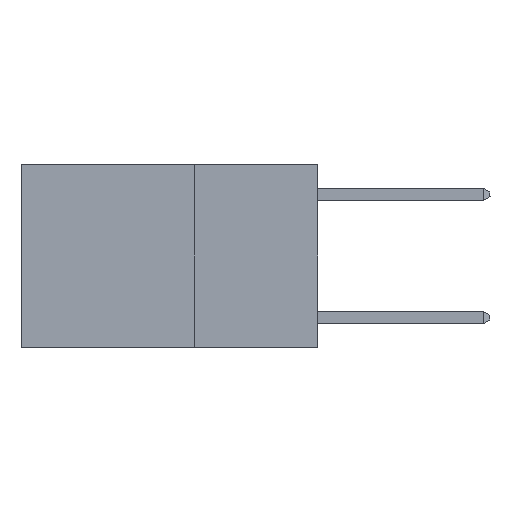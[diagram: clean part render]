
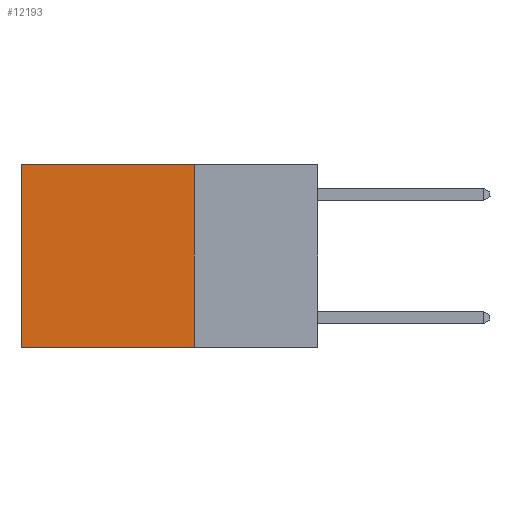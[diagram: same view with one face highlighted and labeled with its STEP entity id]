
A CAD part, left-side view. The second image highlights one B-rep face of the part: STEP entity #12193.
In plain terms, the highlighted planar face has unit normal (-1, 0, 0).
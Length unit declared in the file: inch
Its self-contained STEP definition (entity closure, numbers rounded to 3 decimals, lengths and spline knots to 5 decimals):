
#111 = LINE ( 'NONE', #9162, #2902 ) ;
#251 = VERTEX_POINT ( 'NONE', #11108 ) ;
#793 = CARTESIAN_POINT ( 'NONE',  ( 0.2625, 0.6, -0.37 ) ) ;
#811 = EDGE_CURVE ( 'NONE', #4362, #7198, #11759, .T. ) ;
#1944 = DIRECTION ( 'NONE',  ( 1., 0., 0. ) ) ;
#2175 = VECTOR ( 'NONE', #8121, 39.37008 ) ;
#2902 = VECTOR ( 'NONE', #12830, 39.37008 ) ;
#3704 = CARTESIAN_POINT ( 'NONE',  ( 0.2625, 0.25, -0.37 ) ) ;
#4308 = CARTESIAN_POINT ( 'NONE',  ( 0.2625, 0.25, 0. ) ) ;
#4362 = VERTEX_POINT ( 'NONE', #15962 ) ;
#4978 = LINE ( 'NONE', #3704, #11538 ) ;
#6805 = ORIENTED_EDGE ( 'NONE', *, *, #811, .T. ) ;
#7198 = VERTEX_POINT ( 'NONE', #793 ) ;
#8121 = DIRECTION ( 'NONE',  ( 0., 0., -1. ) ) ;
#8959 = VECTOR ( 'NONE', #14451, 39.37008 ) ;
#9162 = CARTESIAN_POINT ( 'NONE',  ( 0.2625, 0.25, 0. ) ) ;
#9525 = PLANE ( 'NONE',  #11454 ) ;
#9648 = CARTESIAN_POINT ( 'NONE',  ( 0.2625, 0.25, 0. ) ) ;
#10730 = DIRECTION ( 'NONE',  ( 0., 0., -1. ) ) ;
#11108 = CARTESIAN_POINT ( 'NONE',  ( 0.2625, 0.25, -0.37 ) ) ;
#11349 = VERTEX_POINT ( 'NONE', #4308 ) ;
#11454 = AXIS2_PLACEMENT_3D ( 'NONE', #14328, #1944, #10730 ) ;
#11538 = VECTOR ( 'NONE', #13597, 39.37008 ) ;
#11731 = FACE_OUTER_BOUND ( 'NONE', #13338, .T. ) ;
#11759 = LINE ( 'NONE', #14205, #2175 ) ;
#11961 = ORIENTED_EDGE ( 'NONE', *, *, #13583, .T. ) ;
#12193 = ADVANCED_FACE ( 'NONE', ( #11731 ), #9525, .F. ) ;
#12479 = EDGE_CURVE ( 'NONE', #251, #7198, #4978, .T. ) ;
#12830 = DIRECTION ( 'NONE',  ( 0., 1., 0. ) ) ;
#13338 = EDGE_LOOP ( 'NONE', ( #6805, #14043, #14797, #11961 ) ) ;
#13583 = EDGE_CURVE ( 'NONE', #11349, #4362, #111, .T. ) ;
#13597 = DIRECTION ( 'NONE',  ( 0., 1., 0. ) ) ;
#13899 = EDGE_CURVE ( 'NONE', #11349, #251, #15404, .T. ) ;
#14043 = ORIENTED_EDGE ( 'NONE', *, *, #12479, .F. ) ;
#14205 = CARTESIAN_POINT ( 'NONE',  ( 0.2625, 0.6, 0. ) ) ;
#14328 = CARTESIAN_POINT ( 'NONE',  ( 0.2625, 0.25, 0. ) ) ;
#14451 = DIRECTION ( 'NONE',  ( 0., 0., -1. ) ) ;
#14797 = ORIENTED_EDGE ( 'NONE', *, *, #13899, .F. ) ;
#15404 = LINE ( 'NONE', #9648, #8959 ) ;
#15962 = CARTESIAN_POINT ( 'NONE',  ( 0.2625, 0.6, 0. ) ) ;
